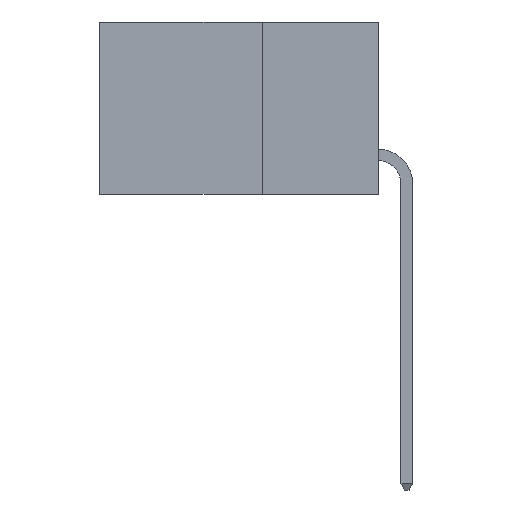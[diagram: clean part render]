
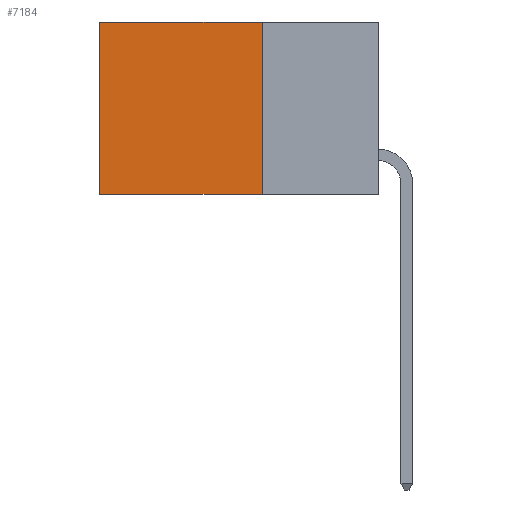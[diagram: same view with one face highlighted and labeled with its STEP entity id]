
A CAD part, left-side view. The second image highlights one B-rep face of the part: STEP entity #7184.
In plain terms, the highlighted planar face has unit normal (-1, 0, 0).
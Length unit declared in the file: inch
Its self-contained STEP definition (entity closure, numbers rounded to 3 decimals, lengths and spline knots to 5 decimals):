
#606 = DIRECTION ( 'NONE',  ( 0., 0., -1. ) ) ;
#755 = LINE ( 'NONE', #10109, #1097 ) ;
#841 = EDGE_LOOP ( 'NONE', ( #3646, #9411, #7448, #7734 ) ) ;
#1097 = VECTOR ( 'NONE', #5026, 39.37008 ) ;
#1137 = LINE ( 'NONE', #9566, #9127 ) ;
#1783 = CARTESIAN_POINT ( 'NONE',  ( 0.2615, 0.6, -0.37 ) ) ;
#2790 = AXIS2_PLACEMENT_3D ( 'NONE', #3813, #6909, #606 ) ;
#2827 = CARTESIAN_POINT ( 'NONE',  ( 0.2615, 0.6, 0. ) ) ;
#3201 = CARTESIAN_POINT ( 'NONE',  ( 0.2615, 0.25, -0.37 ) ) ;
#3646 = ORIENTED_EDGE ( 'NONE', *, *, #10694, .T. ) ;
#3673 = EDGE_CURVE ( 'NONE', #4578, #9187, #1137, .T. ) ;
#3813 = CARTESIAN_POINT ( 'NONE',  ( 0.2615, 0.25, -0.37 ) ) ;
#4578 = VERTEX_POINT ( 'NONE', #4766 ) ;
#4766 = CARTESIAN_POINT ( 'NONE',  ( 0.2615, 0.25, 0. ) ) ;
#4786 = CARTESIAN_POINT ( 'NONE',  ( 0.2615, 0.25, -0.37 ) ) ;
#4905 = EDGE_CURVE ( 'NONE', #9187, #10657, #6096, .T. ) ;
#5026 = DIRECTION ( 'NONE',  ( 0., 0., -1. ) ) ;
#6039 = FACE_OUTER_BOUND ( 'NONE', #841, .T. ) ;
#6096 = LINE ( 'NONE', #3201, #9114 ) ;
#6402 = VECTOR ( 'NONE', #6889, 39.37008 ) ;
#6889 = DIRECTION ( 'NONE',  ( 0., 1., 0. ) ) ;
#6909 = DIRECTION ( 'NONE',  ( 1., 0., 0. ) ) ;
#7184 = ADVANCED_FACE ( 'NONE', ( #6039 ), #7892, .F. ) ;
#7448 = ORIENTED_EDGE ( 'NONE', *, *, #3673, .F. ) ;
#7734 = ORIENTED_EDGE ( 'NONE', *, *, #8548, .T. ) ;
#7892 = PLANE ( 'NONE',  #2790 ) ;
#8548 = EDGE_CURVE ( 'NONE', #4578, #10643, #11529, .T. ) ;
#9114 = VECTOR ( 'NONE', #13463, 39.37008 ) ;
#9127 = VECTOR ( 'NONE', #10595, 39.37008 ) ;
#9187 = VERTEX_POINT ( 'NONE', #4786 ) ;
#9411 = ORIENTED_EDGE ( 'NONE', *, *, #4905, .F. ) ;
#9566 = CARTESIAN_POINT ( 'NONE',  ( 0.2615, 0.25, -0.37 ) ) ;
#9978 = CARTESIAN_POINT ( 'NONE',  ( 0.2615, 0.25, 0. ) ) ;
#10109 = CARTESIAN_POINT ( 'NONE',  ( 0.2615, 0.6, -0.37 ) ) ;
#10595 = DIRECTION ( 'NONE',  ( 0., 0., -1. ) ) ;
#10643 = VERTEX_POINT ( 'NONE', #2827 ) ;
#10657 = VERTEX_POINT ( 'NONE', #1783 ) ;
#10694 = EDGE_CURVE ( 'NONE', #10643, #10657, #755, .T. ) ;
#11529 = LINE ( 'NONE', #9978, #6402 ) ;
#13463 = DIRECTION ( 'NONE',  ( 0., 1., 0. ) ) ;
